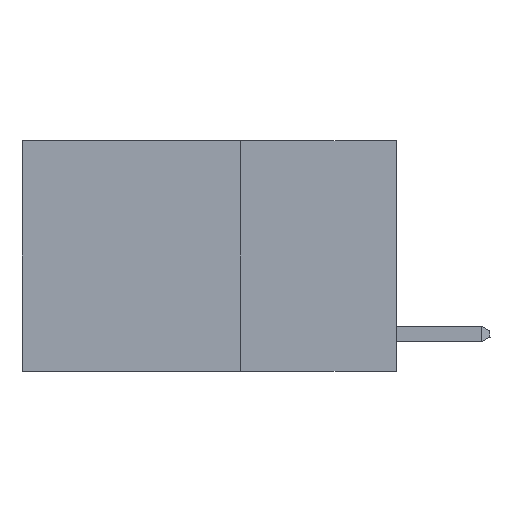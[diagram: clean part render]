
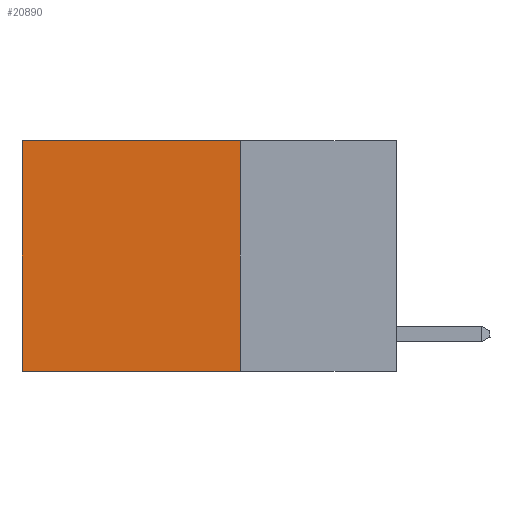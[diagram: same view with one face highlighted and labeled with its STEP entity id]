
A CAD part, left-side view. The second image highlights one B-rep face of the part: STEP entity #20890.
In plain terms, the highlighted planar face has unit normal (-1, 0, 0).
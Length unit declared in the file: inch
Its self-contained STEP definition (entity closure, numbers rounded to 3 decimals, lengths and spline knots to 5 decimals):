
#606 = CARTESIAN_POINT ( 'NONE',  ( 0.2625, 0.25, 0. ) ) ;
#719 = LINE ( 'NONE', #606, #18235 ) ;
#1247 = CARTESIAN_POINT ( 'NONE',  ( 0.2625, 0.25, 0. ) ) ;
#2456 = CARTESIAN_POINT ( 'NONE',  ( 0.2625, 0.6, -0.37 ) ) ;
#2995 = DIRECTION ( 'NONE',  ( 0., 0., -1. ) ) ;
#3101 = DIRECTION ( 'NONE',  ( 1., 0., 0. ) ) ;
#3766 = VERTEX_POINT ( 'NONE', #15782 ) ;
#5811 = DIRECTION ( 'NONE',  ( 0., 1., 0. ) ) ;
#7324 = DIRECTION ( 'NONE',  ( 0., 1., 0. ) ) ;
#9200 = VECTOR ( 'NONE', #17695, 39.37008 ) ;
#9506 = EDGE_CURVE ( 'NONE', #15791, #17125, #13179, .T. ) ;
#9611 = ORIENTED_EDGE ( 'NONE', *, *, #17259, .F. ) ;
#11003 = LINE ( 'NONE', #1247, #9200 ) ;
#11009 = ORIENTED_EDGE ( 'NONE', *, *, #9506, .T. ) ;
#11481 = EDGE_CURVE ( 'NONE', #3766, #15791, #719, .T. ) ;
#11744 = CARTESIAN_POINT ( 'NONE',  ( 0.2625, 0.6, 0. ) ) ;
#11854 = VECTOR ( 'NONE', #19546, 39.37008 ) ;
#13179 = LINE ( 'NONE', #18010, #11854 ) ;
#13502 = ORIENTED_EDGE ( 'NONE', *, *, #11481, .T. ) ;
#14121 = LINE ( 'NONE', #20804, #17526 ) ;
#14186 = EDGE_CURVE ( 'NONE', #20357, #17125, #14121, .T. ) ;
#14603 = FACE_OUTER_BOUND ( 'NONE', #20402, .T. ) ;
#15782 = CARTESIAN_POINT ( 'NONE',  ( 0.2625, 0.25, 0. ) ) ;
#15791 = VERTEX_POINT ( 'NONE', #11744 ) ;
#17125 = VERTEX_POINT ( 'NONE', #2456 ) ;
#17259 = EDGE_CURVE ( 'NONE', #3766, #20357, #11003, .T. ) ;
#17526 = VECTOR ( 'NONE', #5811, 39.37008 ) ;
#17695 = DIRECTION ( 'NONE',  ( 0., 0., -1. ) ) ;
#18010 = CARTESIAN_POINT ( 'NONE',  ( 0.2625, 0.6, 0. ) ) ;
#18235 = VECTOR ( 'NONE', #7324, 39.37008 ) ;
#18708 = AXIS2_PLACEMENT_3D ( 'NONE', #21178, #3101, #2995 ) ;
#18883 = ORIENTED_EDGE ( 'NONE', *, *, #14186, .F. ) ;
#19546 = DIRECTION ( 'NONE',  ( 0., 0., -1. ) ) ;
#19654 = PLANE ( 'NONE',  #18708 ) ;
#20357 = VERTEX_POINT ( 'NONE', #20876 ) ;
#20402 = EDGE_LOOP ( 'NONE', ( #11009, #18883, #9611, #13502 ) ) ;
#20804 = CARTESIAN_POINT ( 'NONE',  ( 0.2625, 0.25, -0.37 ) ) ;
#20876 = CARTESIAN_POINT ( 'NONE',  ( 0.2625, 0.25, -0.37 ) ) ;
#20890 = ADVANCED_FACE ( 'NONE', ( #14603 ), #19654, .F. ) ;
#21178 = CARTESIAN_POINT ( 'NONE',  ( 0.2625, 0.25, 0. ) ) ;
